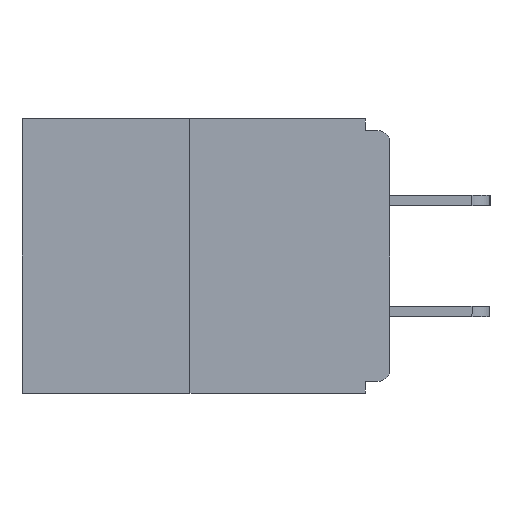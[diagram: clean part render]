
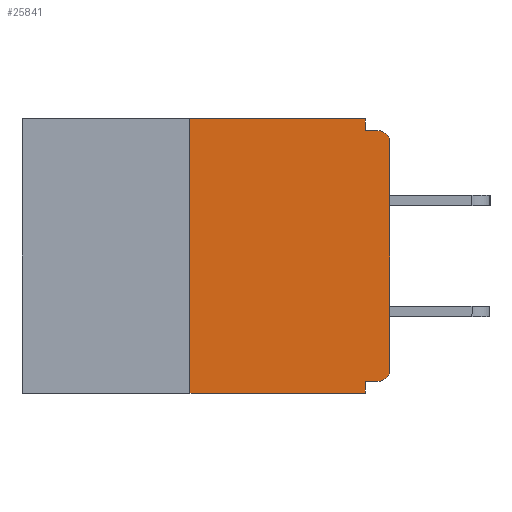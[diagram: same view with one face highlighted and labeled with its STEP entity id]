
A CAD part, left-side view. The second image highlights one B-rep face of the part: STEP entity #25841.
In plain terms, the highlighted planar face has unit normal (-1, 0, 0).
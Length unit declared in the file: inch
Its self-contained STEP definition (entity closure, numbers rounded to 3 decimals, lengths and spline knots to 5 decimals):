
#495 = VERTEX_POINT ( 'NONE', #16481 ) ;
#519 = CARTESIAN_POINT ( 'NONE',  ( 0., 0.031, -0.343 ) ) ;
#705 = DIRECTION ( 'NONE',  ( 0., -1., 0. ) ) ;
#785 = DIRECTION ( 'NONE',  ( -1., 0., 0. ) ) ;
#1112 = DIRECTION ( 'NONE',  ( 1., 0., 0. ) ) ;
#1427 = ORIENTED_EDGE ( 'NONE', *, *, #15715, .F. ) ;
#1969 = VERTEX_POINT ( 'NONE', #12554 ) ;
#2046 = AXIS2_PLACEMENT_3D ( 'NONE', #16768, #785, #16684 ) ;
#2245 = VERTEX_POINT ( 'NONE', #18884 ) ;
#2379 = EDGE_CURVE ( 'NONE', #1969, #10771, #6058, .T. ) ;
#3623 = EDGE_LOOP ( 'NONE', ( #1427, #4252, #6207, #21591, #11961, #24432, #16175, #17330, #8669, #17549 ) ) ;
#4187 = EDGE_CURVE ( 'NONE', #18048, #2245, #22694, .T. ) ;
#4252 = ORIENTED_EDGE ( 'NONE', *, *, #19678, .F. ) ;
#4716 = EDGE_CURVE ( 'NONE', #1969, #15938, #15168, .T. ) ;
#4862 = DIRECTION ( 'NONE',  ( 0., 0., -1. ) ) ;
#5028 = CARTESIAN_POINT ( 'NONE',  ( 0., 0.031, -0.343 ) ) ;
#5354 = PLANE ( 'NONE',  #12693 ) ;
#5442 = VECTOR ( 'NONE', #16984, 39.37008 ) ;
#5561 = DIRECTION ( 'NONE',  ( 0., 0., -1. ) ) ;
#5568 = DIRECTION ( 'NONE',  ( 0., 0., 1. ) ) ;
#5930 = VERTEX_POINT ( 'NONE', #5028 ) ;
#6058 = CIRCLE ( 'NONE', #25742, 0.015 ) ;
#6207 = ORIENTED_EDGE ( 'NONE', *, *, #7896, .T. ) ;
#6340 = CARTESIAN_POINT ( 'NONE',  ( 0., 0., -0.313 ) ) ;
#7158 = CARTESIAN_POINT ( 'NONE',  ( 0., 0.25, 0. ) ) ;
#7619 = DIRECTION ( 'NONE',  ( 0., 0., -1. ) ) ;
#7719 = CARTESIAN_POINT ( 'NONE',  ( 0., 0., -0.015 ) ) ;
#7748 = VECTOR ( 'NONE', #15615, 39.37008 ) ;
#7896 = EDGE_CURVE ( 'NONE', #18674, #5930, #13996, .T. ) ;
#8497 = CARTESIAN_POINT ( 'NONE',  ( 0., 0., -0.03 ) ) ;
#8669 = ORIENTED_EDGE ( 'NONE', *, *, #10883, .F. ) ;
#9656 = CARTESIAN_POINT ( 'NONE',  ( 0., 0., 0. ) ) ;
#10248 = LINE ( 'NONE', #519, #14074 ) ;
#10411 = VECTOR ( 'NONE', #22424, 39.37008 ) ;
#10655 = FACE_OUTER_BOUND ( 'NONE', #3623, .T. ) ;
#10771 = VERTEX_POINT ( 'NONE', #6340 ) ;
#10883 = EDGE_CURVE ( 'NONE', #495, #2245, #14738, .T. ) ;
#11476 = VERTEX_POINT ( 'NONE', #7158 ) ;
#11592 = CARTESIAN_POINT ( 'NONE',  ( 0., 0.031, -0.328 ) ) ;
#11833 = LINE ( 'NONE', #22059, #15943 ) ;
#11914 = EDGE_CURVE ( 'NONE', #15938, #5930, #10248, .T. ) ;
#11961 = ORIENTED_EDGE ( 'NONE', *, *, #4716, .F. ) ;
#12112 = LINE ( 'NONE', #14744, #5442 ) ;
#12554 = CARTESIAN_POINT ( 'NONE',  ( 0., 0.015, -0.328 ) ) ;
#12693 = AXIS2_PLACEMENT_3D ( 'NONE', #23223, #1112, #23323 ) ;
#13996 = LINE ( 'NONE', #18851, #23025 ) ;
#14074 = VECTOR ( 'NONE', #4862, 39.37008 ) ;
#14738 = LINE ( 'NONE', #7719, #7748 ) ;
#14744 = CARTESIAN_POINT ( 'NONE',  ( 0., 0.46, 0. ) ) ;
#14764 = EDGE_CURVE ( 'NONE', #20631, #495, #11833, .T. ) ;
#15168 = LINE ( 'NONE', #22063, #10411 ) ;
#15615 = DIRECTION ( 'NONE',  ( 0., -1., 0. ) ) ;
#15664 = CARTESIAN_POINT ( 'NONE',  ( 0., 0.015, -0.313 ) ) ;
#15715 = EDGE_CURVE ( 'NONE', #11476, #20631, #12112, .T. ) ;
#15938 = VERTEX_POINT ( 'NONE', #11592 ) ;
#15943 = VECTOR ( 'NONE', #7619, 39.37008 ) ;
#15990 = EDGE_CURVE ( 'NONE', #10771, #18048, #20560, .T. ) ;
#16175 = ORIENTED_EDGE ( 'NONE', *, *, #15990, .T. ) ;
#16481 = CARTESIAN_POINT ( 'NONE',  ( 0., 0.031, -0.015 ) ) ;
#16684 = DIRECTION ( 'NONE',  ( 0., 0., -1. ) ) ;
#16768 = CARTESIAN_POINT ( 'NONE',  ( 0., 0.015, -0.03 ) ) ;
#16984 = DIRECTION ( 'NONE',  ( 0., -1., 0. ) ) ;
#17330 = ORIENTED_EDGE ( 'NONE', *, *, #4187, .T. ) ;
#17549 = ORIENTED_EDGE ( 'NONE', *, *, #14764, .F. ) ;
#17566 = VECTOR ( 'NONE', #5568, 39.37008 ) ;
#17865 = LINE ( 'NONE', #23900, #17566 ) ;
#18048 = VERTEX_POINT ( 'NONE', #8497 ) ;
#18674 = VERTEX_POINT ( 'NONE', #21891 ) ;
#18851 = CARTESIAN_POINT ( 'NONE',  ( 0., 0.46, -0.343 ) ) ;
#18884 = CARTESIAN_POINT ( 'NONE',  ( 0., 0.015, -0.015 ) ) ;
#19678 = EDGE_CURVE ( 'NONE', #18674, #11476, #17865, .T. ) ;
#20560 = LINE ( 'NONE', #9656, #24367 ) ;
#20631 = VERTEX_POINT ( 'NONE', #21104 ) ;
#21104 = CARTESIAN_POINT ( 'NONE',  ( 0., 0.031, 0. ) ) ;
#21591 = ORIENTED_EDGE ( 'NONE', *, *, #11914, .F. ) ;
#21891 = CARTESIAN_POINT ( 'NONE',  ( 0., 0.25, -0.343 ) ) ;
#22059 = CARTESIAN_POINT ( 'NONE',  ( 0., 0.031, 0. ) ) ;
#22063 = CARTESIAN_POINT ( 'NONE',  ( 0., 0., -0.328 ) ) ;
#22424 = DIRECTION ( 'NONE',  ( 0., 1., 0. ) ) ;
#22694 = CIRCLE ( 'NONE', #2046, 0.015 ) ;
#23025 = VECTOR ( 'NONE', #705, 39.37008 ) ;
#23223 = CARTESIAN_POINT ( 'NONE',  ( 0., 0.46, 0. ) ) ;
#23323 = DIRECTION ( 'NONE',  ( 0., 0., -1. ) ) ;
#23890 = DIRECTION ( 'NONE',  ( -1., 0., 0. ) ) ;
#23900 = CARTESIAN_POINT ( 'NONE',  ( 0., 0.25, 0. ) ) ;
#23915 = DIRECTION ( 'NONE',  ( 0., 0., 1. ) ) ;
#24367 = VECTOR ( 'NONE', #23915, 39.37008 ) ;
#24432 = ORIENTED_EDGE ( 'NONE', *, *, #2379, .T. ) ;
#25742 = AXIS2_PLACEMENT_3D ( 'NONE', #15664, #23890, #5561 ) ;
#25841 = ADVANCED_FACE ( 'NONE', ( #10655 ), #5354, .F. ) ;
